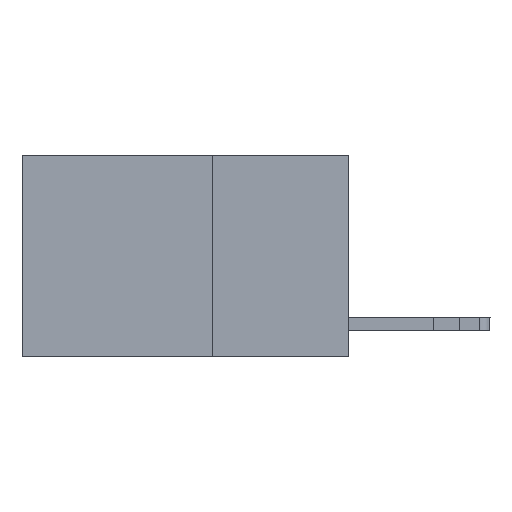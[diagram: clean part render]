
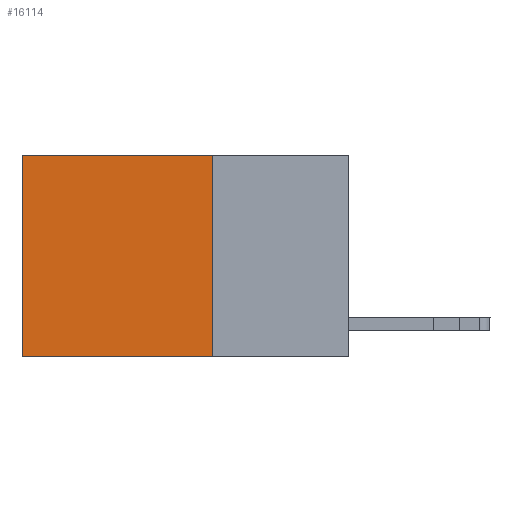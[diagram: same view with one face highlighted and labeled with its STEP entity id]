
A CAD part, left-side view. The second image highlights one B-rep face of the part: STEP entity #16114.
In plain terms, the highlighted planar face has unit normal (-1, 0, 0).
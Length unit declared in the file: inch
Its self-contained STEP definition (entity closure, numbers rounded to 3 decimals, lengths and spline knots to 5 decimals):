
#587 = CARTESIAN_POINT ( 'NONE',  ( 0.2625, 0.25, -0.37 ) ) ;
#1138 = AXIS2_PLACEMENT_3D ( 'NONE', #13523, #6059, #11878 ) ;
#1313 = VERTEX_POINT ( 'NONE', #5935 ) ;
#1599 = EDGE_CURVE ( 'NONE', #15234, #8312, #5636, .T. ) ;
#1794 = EDGE_CURVE ( 'NONE', #1313, #7297, #15972, .T. ) ;
#3331 = VECTOR ( 'NONE', #14531, 39.37008 ) ;
#3903 = CARTESIAN_POINT ( 'NONE',  ( 0.2625, 0.25, 0. ) ) ;
#5547 = CARTESIAN_POINT ( 'NONE',  ( 0.2625, 0.6, 0. ) ) ;
#5636 = LINE ( 'NONE', #5547, #11370 ) ;
#5873 = PLANE ( 'NONE',  #1138 ) ;
#5935 = CARTESIAN_POINT ( 'NONE',  ( 0.2625, 0.25, 0. ) ) ;
#6059 = DIRECTION ( 'NONE',  ( 1., 0., 0. ) ) ;
#6138 = EDGE_LOOP ( 'NONE', ( #12740, #12782, #17013, #9893 ) ) ;
#7297 = VERTEX_POINT ( 'NONE', #11713 ) ;
#7335 = FACE_OUTER_BOUND ( 'NONE', #6138, .T. ) ;
#8171 = LINE ( 'NONE', #3903, #18431 ) ;
#8312 = VERTEX_POINT ( 'NONE', #13520 ) ;
#9893 = ORIENTED_EDGE ( 'NONE', *, *, #13995, .T. ) ;
#10894 = CARTESIAN_POINT ( 'NONE',  ( 0.2625, 0.6, 0. ) ) ;
#11188 = DIRECTION ( 'NONE',  ( 0., 1., 0. ) ) ;
#11370 = VECTOR ( 'NONE', #17017, 39.37008 ) ;
#11713 = CARTESIAN_POINT ( 'NONE',  ( 0.2625, 0.25, -0.37 ) ) ;
#11878 = DIRECTION ( 'NONE',  ( 0., 0., -1. ) ) ;
#12249 = DIRECTION ( 'NONE',  ( 0., 1., 0. ) ) ;
#12740 = ORIENTED_EDGE ( 'NONE', *, *, #1599, .T. ) ;
#12782 = ORIENTED_EDGE ( 'NONE', *, *, #13902, .F. ) ;
#13520 = CARTESIAN_POINT ( 'NONE',  ( 0.2625, 0.6, -0.37 ) ) ;
#13523 = CARTESIAN_POINT ( 'NONE',  ( 0.2625, 0.25, 0. ) ) ;
#13902 = EDGE_CURVE ( 'NONE', #7297, #8312, #14944, .T. ) ;
#13995 = EDGE_CURVE ( 'NONE', #1313, #15234, #8171, .T. ) ;
#14531 = DIRECTION ( 'NONE',  ( 0., 0., -1. ) ) ;
#14944 = LINE ( 'NONE', #587, #17805 ) ;
#15234 = VERTEX_POINT ( 'NONE', #10894 ) ;
#15972 = LINE ( 'NONE', #17603, #3331 ) ;
#16114 = ADVANCED_FACE ( 'NONE', ( #7335 ), #5873, .F. ) ;
#17013 = ORIENTED_EDGE ( 'NONE', *, *, #1794, .F. ) ;
#17017 = DIRECTION ( 'NONE',  ( 0., 0., -1. ) ) ;
#17603 = CARTESIAN_POINT ( 'NONE',  ( 0.2625, 0.25, 0. ) ) ;
#17805 = VECTOR ( 'NONE', #12249, 39.37008 ) ;
#18431 = VECTOR ( 'NONE', #11188, 39.37008 ) ;
